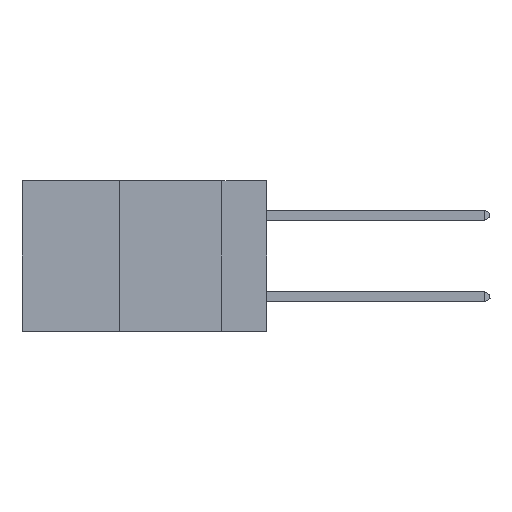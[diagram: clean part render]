
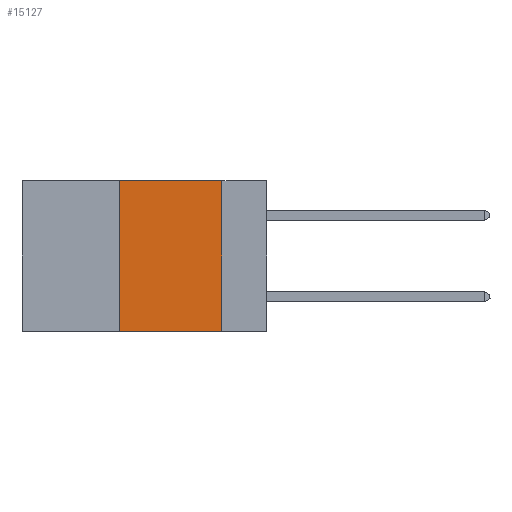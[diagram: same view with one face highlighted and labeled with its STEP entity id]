
A CAD part, left-side view. The second image highlights one B-rep face of the part: STEP entity #15127.
In plain terms, the highlighted planar face has unit normal (-1, 0, 0).
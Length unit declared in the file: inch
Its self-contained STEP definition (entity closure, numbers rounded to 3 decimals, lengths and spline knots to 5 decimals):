
#157 = LINE ( 'NONE', #27478, #7882 ) ;
#436 = VERTEX_POINT ( 'NONE', #12628 ) ;
#2590 = LINE ( 'NONE', #12696, #18509 ) ;
#2653 = DIRECTION ( 'NONE',  ( 0., -1., 0. ) ) ;
#3371 = CARTESIAN_POINT ( 'NONE',  ( 0., 0.36, 0. ) ) ;
#3796 = CARTESIAN_POINT ( 'NONE',  ( 0., 0.11, -0.37 ) ) ;
#4722 = CARTESIAN_POINT ( 'NONE',  ( 0., 0.36, 0. ) ) ;
#6161 = VERTEX_POINT ( 'NONE', #3796 ) ;
#7882 = VECTOR ( 'NONE', #2653, 39.37008 ) ;
#8872 = CARTESIAN_POINT ( 'NONE',  ( 0., 0.11, 0. ) ) ;
#9452 = AXIS2_PLACEMENT_3D ( 'NONE', #19996, #13549, #24865 ) ;
#11373 = ORIENTED_EDGE ( 'NONE', *, *, #18119, .F. ) ;
#12628 = CARTESIAN_POINT ( 'NONE',  ( 0., 0.11, 0. ) ) ;
#12696 = CARTESIAN_POINT ( 'NONE',  ( 0., 0.6, -0.37 ) ) ;
#13549 = DIRECTION ( 'NONE',  ( 1., 0., 0. ) ) ;
#15127 = ADVANCED_FACE ( 'NONE', ( #24623 ), #26829, .F. ) ;
#16257 = VECTOR ( 'NONE', #25948, 39.37008 ) ;
#17476 = CARTESIAN_POINT ( 'NONE',  ( 0., 0.36, -0.37 ) ) ;
#18119 = EDGE_CURVE ( 'NONE', #22634, #23448, #27929, .T. ) ;
#18509 = VECTOR ( 'NONE', #25998, 39.37008 ) ;
#19821 = EDGE_LOOP ( 'NONE', ( #22361, #20229, #11373, #28547 ) ) ;
#19996 = CARTESIAN_POINT ( 'NONE',  ( 0., 0.6, 0. ) ) ;
#20229 = ORIENTED_EDGE ( 'NONE', *, *, #27965, .F. ) ;
#21643 = LINE ( 'NONE', #8872, #24495 ) ;
#22361 = ORIENTED_EDGE ( 'NONE', *, *, #24731, .F. ) ;
#22634 = VERTEX_POINT ( 'NONE', #17476 ) ;
#23448 = VERTEX_POINT ( 'NONE', #4722 ) ;
#23702 = EDGE_CURVE ( 'NONE', #22634, #6161, #2590, .T. ) ;
#24495 = VECTOR ( 'NONE', #24776, 39.37008 ) ;
#24623 = FACE_OUTER_BOUND ( 'NONE', #19821, .T. ) ;
#24731 = EDGE_CURVE ( 'NONE', #436, #6161, #21643, .T. ) ;
#24776 = DIRECTION ( 'NONE',  ( 0., 0., -1. ) ) ;
#24865 = DIRECTION ( 'NONE',  ( 0., 0., -1. ) ) ;
#25948 = DIRECTION ( 'NONE',  ( 0., 0., 1. ) ) ;
#25998 = DIRECTION ( 'NONE',  ( 0., -1., 0. ) ) ;
#26829 = PLANE ( 'NONE',  #9452 ) ;
#27478 = CARTESIAN_POINT ( 'NONE',  ( 0., 0.6, 0. ) ) ;
#27929 = LINE ( 'NONE', #3371, #16257 ) ;
#27965 = EDGE_CURVE ( 'NONE', #23448, #436, #157, .T. ) ;
#28547 = ORIENTED_EDGE ( 'NONE', *, *, #23702, .T. ) ;
